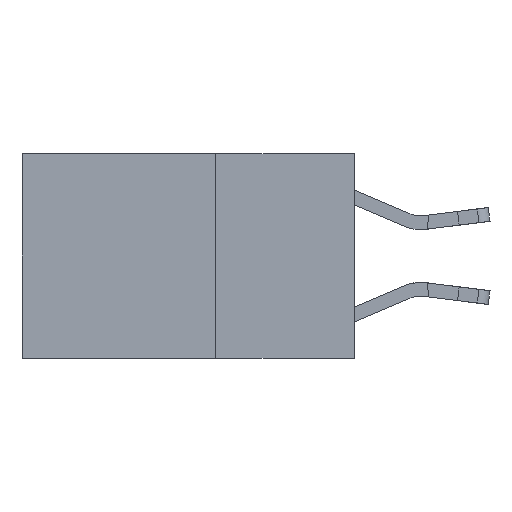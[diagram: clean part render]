
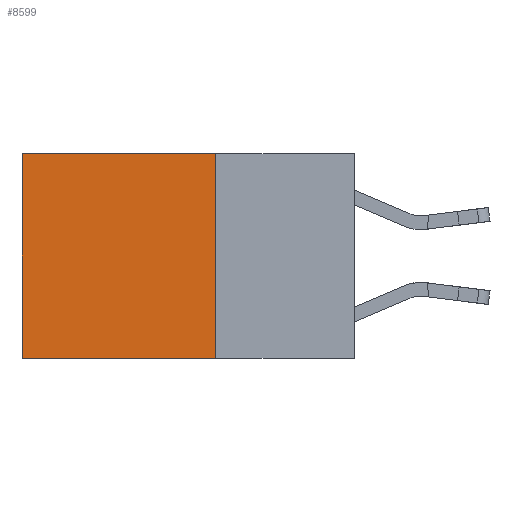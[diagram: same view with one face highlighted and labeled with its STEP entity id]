
A CAD part, left-side view. The second image highlights one B-rep face of the part: STEP entity #8599.
In plain terms, the highlighted planar face has unit normal (-1, 0, 0).
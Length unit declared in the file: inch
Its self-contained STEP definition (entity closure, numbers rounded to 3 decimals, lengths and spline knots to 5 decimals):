
#394 = CARTESIAN_POINT ( 'NONE',  ( 0.2625, 0.6, -0.37 ) ) ;
#1930 = CARTESIAN_POINT ( 'NONE',  ( 0.2625, 0.25, -0.37 ) ) ;
#4443 = VECTOR ( 'NONE', #5598, 39.37008 ) ;
#4975 = PLANE ( 'NONE',  #13993 ) ;
#5598 = DIRECTION ( 'NONE',  ( 0., 0., -1. ) ) ;
#5849 = CARTESIAN_POINT ( 'NONE',  ( 0.2625, 0.25, 0. ) ) ;
#7004 = LINE ( 'NONE', #8830, #17756 ) ;
#7070 = VERTEX_POINT ( 'NONE', #394 ) ;
#7289 = CARTESIAN_POINT ( 'NONE',  ( 0.2625, 0.25, 0. ) ) ;
#8126 = LINE ( 'NONE', #21845, #12067 ) ;
#8135 = ORIENTED_EDGE ( 'NONE', *, *, #13933, .F. ) ;
#8599 = ADVANCED_FACE ( 'NONE', ( #22827 ), #4975, .F. ) ;
#8830 = CARTESIAN_POINT ( 'NONE',  ( 0.2625, 0.6, 0. ) ) ;
#8910 = EDGE_CURVE ( 'NONE', #22804, #7070, #7004, .T. ) ;
#9674 = VERTEX_POINT ( 'NONE', #1930 ) ;
#10180 = DIRECTION ( 'NONE',  ( 0., 1., 0. ) ) ;
#10515 = EDGE_CURVE ( 'NONE', #13634, #9674, #23197, .T. ) ;
#11151 = DIRECTION ( 'NONE',  ( 1., 0., 0. ) ) ;
#12067 = VECTOR ( 'NONE', #10180, 39.37008 ) ;
#13634 = VERTEX_POINT ( 'NONE', #18944 ) ;
#13933 = EDGE_CURVE ( 'NONE', #9674, #7070, #8126, .T. ) ;
#13993 = AXIS2_PLACEMENT_3D ( 'NONE', #7289, #11151, #21153 ) ;
#16617 = DIRECTION ( 'NONE',  ( 0., 0., -1. ) ) ;
#17756 = VECTOR ( 'NONE', #16617, 39.37008 ) ;
#18541 = CARTESIAN_POINT ( 'NONE',  ( 0.2625, 0.25, 0. ) ) ;
#18548 = ORIENTED_EDGE ( 'NONE', *, *, #24534, .T. ) ;
#18944 = CARTESIAN_POINT ( 'NONE',  ( 0.2625, 0.25, 0. ) ) ;
#20025 = ORIENTED_EDGE ( 'NONE', *, *, #8910, .T. ) ;
#20156 = EDGE_LOOP ( 'NONE', ( #20025, #8135, #23198, #18548 ) ) ;
#20471 = LINE ( 'NONE', #18541, #20502 ) ;
#20502 = VECTOR ( 'NONE', #24467, 39.37008 ) ;
#21153 = DIRECTION ( 'NONE',  ( 0., 0., -1. ) ) ;
#21845 = CARTESIAN_POINT ( 'NONE',  ( 0.2625, 0.25, -0.37 ) ) ;
#22804 = VERTEX_POINT ( 'NONE', #24099 ) ;
#22827 = FACE_OUTER_BOUND ( 'NONE', #20156, .T. ) ;
#23197 = LINE ( 'NONE', #5849, #4443 ) ;
#23198 = ORIENTED_EDGE ( 'NONE', *, *, #10515, .F. ) ;
#24099 = CARTESIAN_POINT ( 'NONE',  ( 0.2625, 0.6, 0. ) ) ;
#24467 = DIRECTION ( 'NONE',  ( 0., 1., 0. ) ) ;
#24534 = EDGE_CURVE ( 'NONE', #13634, #22804, #20471, .T. ) ;
